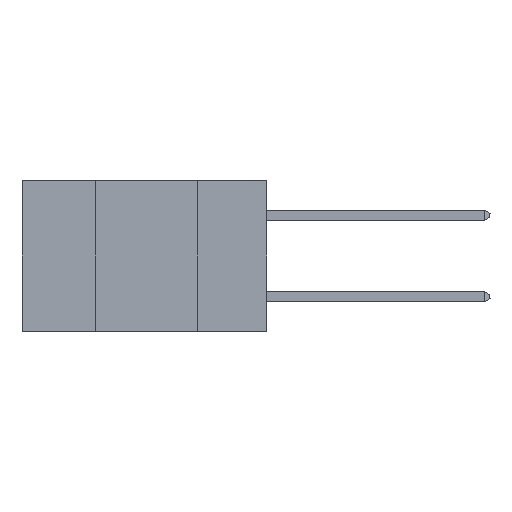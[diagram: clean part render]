
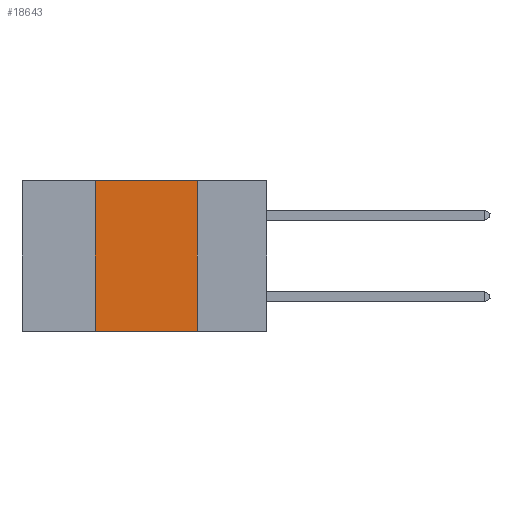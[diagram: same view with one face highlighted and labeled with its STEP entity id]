
A CAD part, left-side view. The second image highlights one B-rep face of the part: STEP entity #18643.
In plain terms, the highlighted planar face has unit normal (-1, 0, 0).
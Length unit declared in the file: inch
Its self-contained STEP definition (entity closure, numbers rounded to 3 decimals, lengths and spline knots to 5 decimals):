
#14 = DIRECTION ( 'NONE',  ( 0., 0., -1. ) ) ;
#141 = DIRECTION ( 'NONE',  ( 0., 0., -1. ) ) ;
#2768 = FACE_OUTER_BOUND ( 'NONE', #20136, .T. ) ;
#3765 = ORIENTED_EDGE ( 'NONE', *, *, #4933, .T. ) ;
#4305 = DIRECTION ( 'NONE',  ( 0., 0., 1. ) ) ;
#4933 = EDGE_CURVE ( 'NONE', #27279, #12640, #12318, .T. ) ;
#6042 = CARTESIAN_POINT ( 'NONE',  ( 0., 0.42, 0. ) ) ;
#6446 = VERTEX_POINT ( 'NONE', #23635 ) ;
#6757 = CARTESIAN_POINT ( 'NONE',  ( 0., 0.17, -0.37 ) ) ;
#7143 = LINE ( 'NONE', #13141, #16359 ) ;
#7412 = EDGE_CURVE ( 'NONE', #23710, #6446, #7143, .T. ) ;
#8058 = EDGE_CURVE ( 'NONE', #6446, #12640, #19471, .T. ) ;
#9444 = AXIS2_PLACEMENT_3D ( 'NONE', #25331, #30800, #141 ) ;
#10577 = DIRECTION ( 'NONE',  ( 0., -1., 0. ) ) ;
#10671 = EDGE_CURVE ( 'NONE', #27279, #23710, #22538, .T. ) ;
#12318 = LINE ( 'NONE', #25865, #30312 ) ;
#12452 = CARTESIAN_POINT ( 'NONE',  ( 0., 0.17, 0. ) ) ;
#12640 = VERTEX_POINT ( 'NONE', #6757 ) ;
#13141 = CARTESIAN_POINT ( 'NONE',  ( 0., 0.6, 0. ) ) ;
#14168 = ORIENTED_EDGE ( 'NONE', *, *, #10671, .F. ) ;
#16359 = VECTOR ( 'NONE', #22679, 39.37008 ) ;
#18643 = ADVANCED_FACE ( 'NONE', ( #2768 ), #20215, .F. ) ;
#19471 = LINE ( 'NONE', #12452, #32285 ) ;
#20136 = EDGE_LOOP ( 'NONE', ( #31346, #25076, #14168, #3765 ) ) ;
#20215 = PLANE ( 'NONE',  #9444 ) ;
#21284 = VECTOR ( 'NONE', #4305, 39.37008 ) ;
#22020 = CARTESIAN_POINT ( 'NONE',  ( 0., 0.42, -0.37 ) ) ;
#22538 = LINE ( 'NONE', #27224, #21284 ) ;
#22679 = DIRECTION ( 'NONE',  ( 0., -1., 0. ) ) ;
#23635 = CARTESIAN_POINT ( 'NONE',  ( 0., 0.17, 0. ) ) ;
#23710 = VERTEX_POINT ( 'NONE', #6042 ) ;
#25076 = ORIENTED_EDGE ( 'NONE', *, *, #7412, .F. ) ;
#25331 = CARTESIAN_POINT ( 'NONE',  ( 0., 0.6, 0. ) ) ;
#25865 = CARTESIAN_POINT ( 'NONE',  ( 0., 0.6, -0.37 ) ) ;
#27224 = CARTESIAN_POINT ( 'NONE',  ( 0., 0.42, 0. ) ) ;
#27279 = VERTEX_POINT ( 'NONE', #22020 ) ;
#30312 = VECTOR ( 'NONE', #10577, 39.37008 ) ;
#30800 = DIRECTION ( 'NONE',  ( 1., 0., 0. ) ) ;
#31346 = ORIENTED_EDGE ( 'NONE', *, *, #8058, .F. ) ;
#32285 = VECTOR ( 'NONE', #14, 39.37008 ) ;
